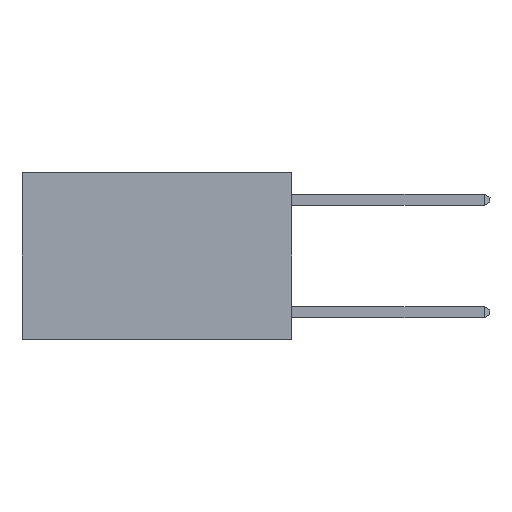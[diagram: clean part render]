
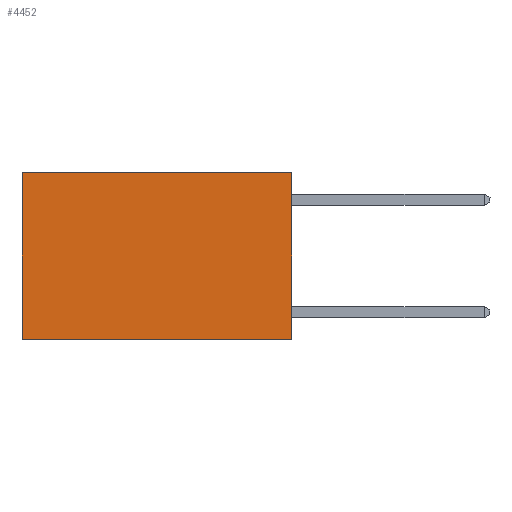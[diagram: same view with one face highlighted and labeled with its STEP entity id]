
A CAD part, left-side view. The second image highlights one B-rep face of the part: STEP entity #4452.
In plain terms, the highlighted planar face has unit normal (-1, 0, 0).
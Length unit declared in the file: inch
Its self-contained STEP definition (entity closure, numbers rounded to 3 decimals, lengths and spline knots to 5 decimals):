
#72 = DIRECTION ( 'NONE',  ( 0., 1., 0. ) ) ;
#945 = VERTEX_POINT ( 'NONE', #3662 ) ;
#976 = VERTEX_POINT ( 'NONE', #3496 ) ;
#1385 = FACE_OUTER_BOUND ( 'NONE', #3372, .T. ) ;
#1735 = ORIENTED_EDGE ( 'NONE', *, *, #6708, .F. ) ;
#1812 = VERTEX_POINT ( 'NONE', #4093 ) ;
#1973 = VECTOR ( 'NONE', #5723, 39.37008 ) ;
#2003 = CARTESIAN_POINT ( 'NONE',  ( 0.2625, 0., 0. ) ) ;
#3372 = EDGE_LOOP ( 'NONE', ( #7499, #1735, #3663, #5814 ) ) ;
#3496 = CARTESIAN_POINT ( 'NONE',  ( 0.2625, 0.6, -0.37 ) ) ;
#3509 = DIRECTION ( 'NONE',  ( 0., 1., 0. ) ) ;
#3548 = LINE ( 'NONE', #5141, #7399 ) ;
#3662 = CARTESIAN_POINT ( 'NONE',  ( 0.2625, 0., 0. ) ) ;
#3663 = ORIENTED_EDGE ( 'NONE', *, *, #8819, .F. ) ;
#4093 = CARTESIAN_POINT ( 'NONE',  ( 0.2625, 0., -0.37 ) ) ;
#4299 = DIRECTION ( 'NONE',  ( 0., 0., -1. ) ) ;
#4385 = VECTOR ( 'NONE', #72, 39.37008 ) ;
#4452 = ADVANCED_FACE ( 'NONE', ( #1385 ), #8035, .F. ) ;
#4643 = DIRECTION ( 'NONE',  ( 0., 0., -1. ) ) ;
#4689 = EDGE_CURVE ( 'NONE', #4757, #976, #6303, .T. ) ;
#4757 = VERTEX_POINT ( 'NONE', #5842 ) ;
#4871 = VECTOR ( 'NONE', #4643, 39.37008 ) ;
#4881 = AXIS2_PLACEMENT_3D ( 'NONE', #2003, #8745, #4299 ) ;
#5108 = EDGE_CURVE ( 'NONE', #945, #4757, #3548, .T. ) ;
#5141 = CARTESIAN_POINT ( 'NONE',  ( 0.2625, 0., 0. ) ) ;
#5723 = DIRECTION ( 'NONE',  ( 0., 0., -1. ) ) ;
#5814 = ORIENTED_EDGE ( 'NONE', *, *, #5108, .T. ) ;
#5842 = CARTESIAN_POINT ( 'NONE',  ( 0.2625, 0.6, 0. ) ) ;
#6303 = LINE ( 'NONE', #7860, #1973 ) ;
#6708 = EDGE_CURVE ( 'NONE', #1812, #976, #6918, .T. ) ;
#6879 = LINE ( 'NONE', #8329, #4871 ) ;
#6918 = LINE ( 'NONE', #8940, #4385 ) ;
#7399 = VECTOR ( 'NONE', #3509, 39.37008 ) ;
#7499 = ORIENTED_EDGE ( 'NONE', *, *, #4689, .T. ) ;
#7860 = CARTESIAN_POINT ( 'NONE',  ( 0.2625, 0.6, 0. ) ) ;
#8035 = PLANE ( 'NONE',  #4881 ) ;
#8329 = CARTESIAN_POINT ( 'NONE',  ( 0.2625, 0., 0. ) ) ;
#8745 = DIRECTION ( 'NONE',  ( 1., 0., 0. ) ) ;
#8819 = EDGE_CURVE ( 'NONE', #945, #1812, #6879, .T. ) ;
#8940 = CARTESIAN_POINT ( 'NONE',  ( 0.2625, 0., -0.37 ) ) ;
